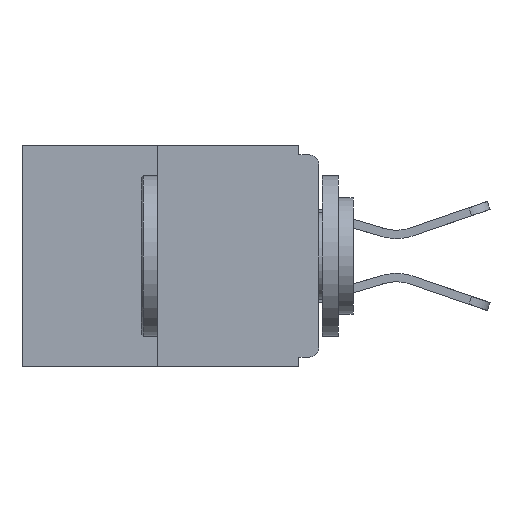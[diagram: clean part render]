
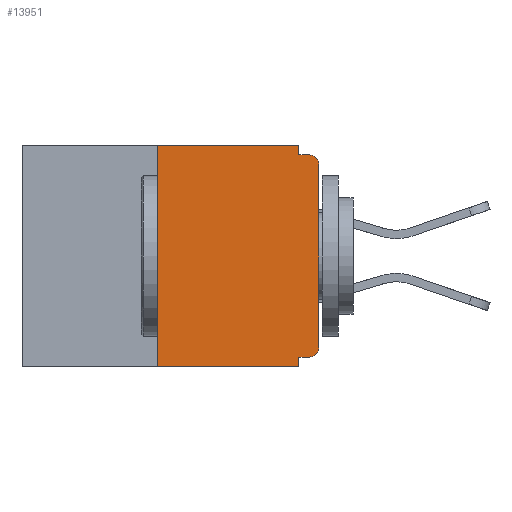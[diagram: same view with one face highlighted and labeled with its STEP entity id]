
A CAD part, left-side view. The second image highlights one B-rep face of the part: STEP entity #13951.
In plain terms, the highlighted planar face has unit normal (-1, 0, 0).
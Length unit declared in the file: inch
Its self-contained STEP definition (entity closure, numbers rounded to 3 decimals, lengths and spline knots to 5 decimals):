
#99 = FACE_OUTER_BOUND ( 'NONE', #15494, .T. ) ;
#521 = ORIENTED_EDGE ( 'NONE', *, *, #15545, .T. ) ;
#685 = CARTESIAN_POINT ( 'NONE',  ( 0., 0., -0.313 ) ) ;
#695 = DIRECTION ( 'NONE',  ( 0., 0., -1. ) ) ;
#950 = ORIENTED_EDGE ( 'NONE', *, *, #15506, .F. ) ;
#1475 = CIRCLE ( 'NONE', #8680, 0.015 ) ;
#1611 = ORIENTED_EDGE ( 'NONE', *, *, #6848, .T. ) ;
#1645 = EDGE_CURVE ( 'NONE', #2054, #15326, #10500, .T. ) ;
#1860 = VECTOR ( 'NONE', #16400, 39.37008 ) ;
#2054 = VERTEX_POINT ( 'NONE', #13923 ) ;
#2087 = CARTESIAN_POINT ( 'NONE',  ( 0., 0., -0.328 ) ) ;
#2312 = VERTEX_POINT ( 'NONE', #11786 ) ;
#2456 = LINE ( 'NONE', #15889, #11769 ) ;
#2923 = AXIS2_PLACEMENT_3D ( 'NONE', #15121, #16393, #15177 ) ;
#3144 = EDGE_CURVE ( 'NONE', #2312, #5585, #3931, .T. ) ;
#3283 = CARTESIAN_POINT ( 'NONE',  ( 0., 0.46, -0.343 ) ) ;
#3697 = CARTESIAN_POINT ( 'NONE',  ( 0., 0.015, -0.015 ) ) ;
#3726 = DIRECTION ( 'NONE',  ( 0., 0., 1. ) ) ;
#3931 = LINE ( 'NONE', #2087, #12892 ) ;
#4224 = ORIENTED_EDGE ( 'NONE', *, *, #8823, .F. ) ;
#4362 = ORIENTED_EDGE ( 'NONE', *, *, #1645, .F. ) ;
#4402 = DIRECTION ( 'NONE',  ( 0., -1., 0. ) ) ;
#4438 = EDGE_CURVE ( 'NONE', #13203, #5994, #12601, .T. ) ;
#4456 = VECTOR ( 'NONE', #3726, 39.37008 ) ;
#4765 = EDGE_CURVE ( 'NONE', #10171, #2054, #13188, .T. ) ;
#4983 = PLANE ( 'NONE',  #2923 ) ;
#5152 = CARTESIAN_POINT ( 'NONE',  ( 0., 0.25, 0. ) ) ;
#5223 = CARTESIAN_POINT ( 'NONE',  ( 0., 0.015, -0.03 ) ) ;
#5365 = ORIENTED_EDGE ( 'NONE', *, *, #14428, .T. ) ;
#5585 = VERTEX_POINT ( 'NONE', #11169 ) ;
#5994 = VERTEX_POINT ( 'NONE', #11395 ) ;
#6159 = EDGE_CURVE ( 'NONE', #12331, #12744, #9745, .T. ) ;
#6244 = ORIENTED_EDGE ( 'NONE', *, *, #4765, .F. ) ;
#6848 = EDGE_CURVE ( 'NONE', #12331, #13952, #10322, .T. ) ;
#7406 = CARTESIAN_POINT ( 'NONE',  ( 0., 0., -0.015 ) ) ;
#7464 = CARTESIAN_POINT ( 'NONE',  ( 0., 0.031, 0. ) ) ;
#7682 = CARTESIAN_POINT ( 'NONE',  ( 0., 0.031, -0.343 ) ) ;
#7774 = DIRECTION ( 'NONE',  ( -1., 0., 0. ) ) ;
#8680 = AXIS2_PLACEMENT_3D ( 'NONE', #5223, #7774, #8960 ) ;
#8753 = VECTOR ( 'NONE', #4402, 39.37008 ) ;
#8812 = CIRCLE ( 'NONE', #9408, 0.015 ) ;
#8823 = EDGE_CURVE ( 'NONE', #12744, #10171, #14827, .T. ) ;
#8960 = DIRECTION ( 'NONE',  ( 0., 0., -1. ) ) ;
#9351 = DIRECTION ( 'NONE',  ( -1., 0., 0. ) ) ;
#9408 = AXIS2_PLACEMENT_3D ( 'NONE', #13191, #9351, #14500 ) ;
#9441 = VECTOR ( 'NONE', #15658, 39.37008 ) ;
#9697 = ORIENTED_EDGE ( 'NONE', *, *, #4438, .T. ) ;
#9745 = LINE ( 'NONE', #5152, #12753 ) ;
#10171 = VERTEX_POINT ( 'NONE', #13390 ) ;
#10322 = LINE ( 'NONE', #3283, #8753 ) ;
#10500 = LINE ( 'NONE', #7406, #10917 ) ;
#10917 = VECTOR ( 'NONE', #15182, 39.37008 ) ;
#11011 = CARTESIAN_POINT ( 'NONE',  ( 0., 0.25, 0. ) ) ;
#11169 = CARTESIAN_POINT ( 'NONE',  ( 0., 0.031, -0.328 ) ) ;
#11395 = CARTESIAN_POINT ( 'NONE',  ( 0., 0., -0.03 ) ) ;
#11647 = CARTESIAN_POINT ( 'NONE',  ( 0., 0.25, -0.343 ) ) ;
#11769 = VECTOR ( 'NONE', #695, 39.37008 ) ;
#11786 = CARTESIAN_POINT ( 'NONE',  ( 0., 0.015, -0.328 ) ) ;
#12331 = VERTEX_POINT ( 'NONE', #11647 ) ;
#12601 = LINE ( 'NONE', #13840, #4456 ) ;
#12744 = VERTEX_POINT ( 'NONE', #11011 ) ;
#12753 = VECTOR ( 'NONE', #14046, 39.37008 ) ;
#12892 = VECTOR ( 'NONE', #15997, 39.37008 ) ;
#13188 = LINE ( 'NONE', #7464, #1860 ) ;
#13191 = CARTESIAN_POINT ( 'NONE',  ( 0., 0.015, -0.313 ) ) ;
#13203 = VERTEX_POINT ( 'NONE', #685 ) ;
#13390 = CARTESIAN_POINT ( 'NONE',  ( 0., 0.031, 0. ) ) ;
#13840 = CARTESIAN_POINT ( 'NONE',  ( 0., 0., 0. ) ) ;
#13923 = CARTESIAN_POINT ( 'NONE',  ( 0., 0.031, -0.015 ) ) ;
#13951 = ADVANCED_FACE ( 'NONE', ( #99 ), #4983, .F. ) ;
#13952 = VERTEX_POINT ( 'NONE', #7682 ) ;
#14046 = DIRECTION ( 'NONE',  ( 0., 0., 1. ) ) ;
#14428 = EDGE_CURVE ( 'NONE', #5994, #15326, #1475, .T. ) ;
#14500 = DIRECTION ( 'NONE',  ( 0., 0., -1. ) ) ;
#14505 = ORIENTED_EDGE ( 'NONE', *, *, #3144, .F. ) ;
#14827 = LINE ( 'NONE', #15607, #9441 ) ;
#15121 = CARTESIAN_POINT ( 'NONE',  ( 0., 0.46, 0. ) ) ;
#15177 = DIRECTION ( 'NONE',  ( 0., 0., -1. ) ) ;
#15182 = DIRECTION ( 'NONE',  ( 0., -1., 0. ) ) ;
#15326 = VERTEX_POINT ( 'NONE', #3697 ) ;
#15494 = EDGE_LOOP ( 'NONE', ( #4224, #16427, #1611, #950, #14505, #521, #9697, #5365, #4362, #6244 ) ) ;
#15506 = EDGE_CURVE ( 'NONE', #5585, #13952, #2456, .T. ) ;
#15545 = EDGE_CURVE ( 'NONE', #2312, #13203, #8812, .T. ) ;
#15607 = CARTESIAN_POINT ( 'NONE',  ( 0., 0.46, 0. ) ) ;
#15658 = DIRECTION ( 'NONE',  ( 0., -1., 0. ) ) ;
#15889 = CARTESIAN_POINT ( 'NONE',  ( 0., 0.031, -0.343 ) ) ;
#15997 = DIRECTION ( 'NONE',  ( 0., 1., 0. ) ) ;
#16393 = DIRECTION ( 'NONE',  ( 1., 0., 0. ) ) ;
#16400 = DIRECTION ( 'NONE',  ( 0., 0., -1. ) ) ;
#16427 = ORIENTED_EDGE ( 'NONE', *, *, #6159, .F. ) ;
